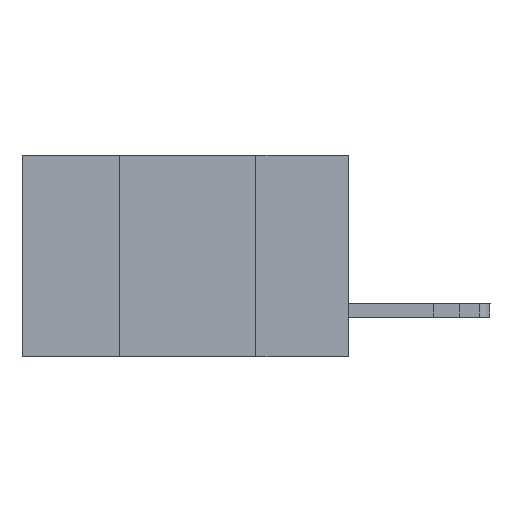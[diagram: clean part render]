
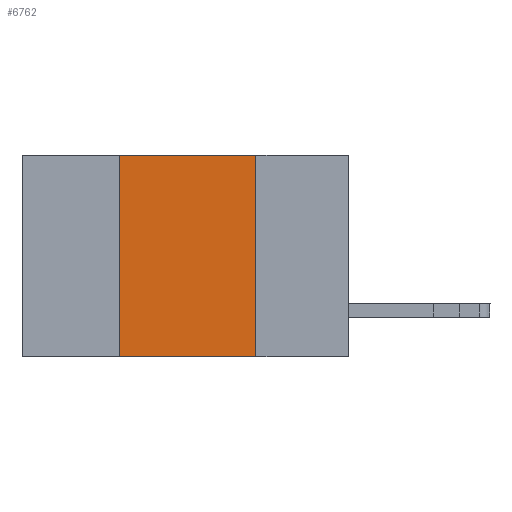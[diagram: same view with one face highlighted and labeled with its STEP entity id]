
A CAD part, left-side view. The second image highlights one B-rep face of the part: STEP entity #6762.
In plain terms, the highlighted planar face has unit normal (-1, 0, 0).
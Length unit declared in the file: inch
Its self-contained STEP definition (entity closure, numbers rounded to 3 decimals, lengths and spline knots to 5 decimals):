
#163 = VECTOR ( 'NONE', #12897, 39.37008 ) ;
#355 = CARTESIAN_POINT ( 'NONE',  ( 0., 0.17, -0.37 ) ) ;
#441 = PLANE ( 'NONE',  #11787 ) ;
#1544 = CARTESIAN_POINT ( 'NONE',  ( 0., 0.42, -0.37 ) ) ;
#1813 = CARTESIAN_POINT ( 'NONE',  ( 0., 0.6, 0. ) ) ;
#1972 = ORIENTED_EDGE ( 'NONE', *, *, #5591, .T. ) ;
#2556 = VERTEX_POINT ( 'NONE', #8567 ) ;
#4263 = LINE ( 'NONE', #13197, #163 ) ;
#4961 = EDGE_CURVE ( 'NONE', #2556, #5029, #6216, .T. ) ;
#5029 = VERTEX_POINT ( 'NONE', #8251 ) ;
#5591 = EDGE_CURVE ( 'NONE', #8459, #5029, #4263, .T. ) ;
#6204 = VERTEX_POINT ( 'NONE', #13097 ) ;
#6216 = LINE ( 'NONE', #355, #10229 ) ;
#6558 = EDGE_LOOP ( 'NONE', ( #13179, #9178, #16753, #1972 ) ) ;
#6762 = ADVANCED_FACE ( 'NONE', ( #18546 ), #441, .F. ) ;
#7113 = VECTOR ( 'NONE', #10645, 39.37008 ) ;
#7145 = DIRECTION ( 'NONE',  ( 0., 0., -1. ) ) ;
#8170 = CARTESIAN_POINT ( 'NONE',  ( 0., 0.6, 0. ) ) ;
#8251 = CARTESIAN_POINT ( 'NONE',  ( 0., 0.17, -0.37 ) ) ;
#8301 = VECTOR ( 'NONE', #13913, 39.37008 ) ;
#8459 = VERTEX_POINT ( 'NONE', #14522 ) ;
#8551 = DIRECTION ( 'NONE',  ( 0., 0., -1. ) ) ;
#8567 = CARTESIAN_POINT ( 'NONE',  ( 0., 0.17, 0. ) ) ;
#9178 = ORIENTED_EDGE ( 'NONE', *, *, #13482, .F. ) ;
#10229 = VECTOR ( 'NONE', #7145, 39.37008 ) ;
#10645 = DIRECTION ( 'NONE',  ( 0., 0., 1. ) ) ;
#11014 = LINE ( 'NONE', #1544, #7113 ) ;
#11787 = AXIS2_PLACEMENT_3D ( 'NONE', #1813, #15190, #8551 ) ;
#12113 = LINE ( 'NONE', #8170, #8301 ) ;
#12897 = DIRECTION ( 'NONE',  ( 0., -1., 0. ) ) ;
#13097 = CARTESIAN_POINT ( 'NONE',  ( 0., 0.42, 0. ) ) ;
#13179 = ORIENTED_EDGE ( 'NONE', *, *, #4961, .F. ) ;
#13197 = CARTESIAN_POINT ( 'NONE',  ( 0., 0.6, -0.37 ) ) ;
#13482 = EDGE_CURVE ( 'NONE', #6204, #2556, #12113, .T. ) ;
#13913 = DIRECTION ( 'NONE',  ( 0., -1., 0. ) ) ;
#14522 = CARTESIAN_POINT ( 'NONE',  ( 0., 0.42, -0.37 ) ) ;
#15190 = DIRECTION ( 'NONE',  ( 1., 0., 0. ) ) ;
#15402 = EDGE_CURVE ( 'NONE', #8459, #6204, #11014, .T. ) ;
#16753 = ORIENTED_EDGE ( 'NONE', *, *, #15402, .F. ) ;
#18546 = FACE_OUTER_BOUND ( 'NONE', #6558, .T. ) ;
